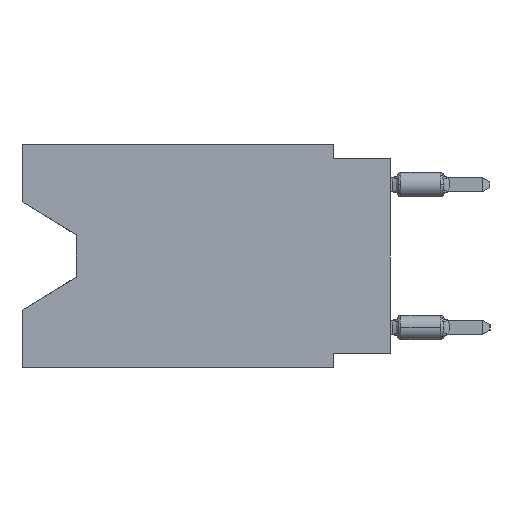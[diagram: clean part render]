
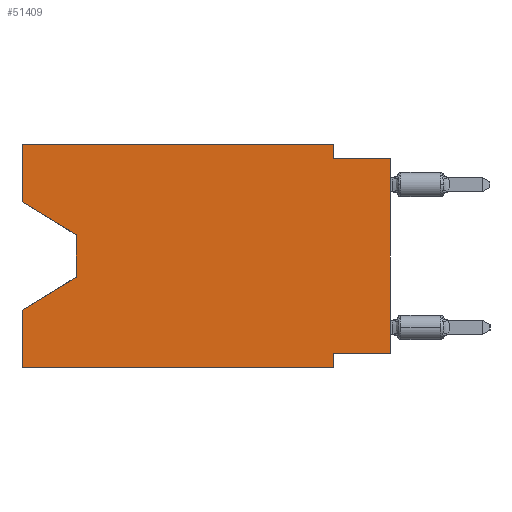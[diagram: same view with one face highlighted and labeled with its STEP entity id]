
A CAD part, left-side view. The second image highlights one B-rep face of the part: STEP entity #51409.
In plain terms, the highlighted planar face has unit normal (-1, 0, 0).
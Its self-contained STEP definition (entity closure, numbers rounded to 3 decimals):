
#362 = CARTESIAN_POINT ( 'NONE',  ( 0., 2.54, 0. ) ) ;
#564 = CARTESIAN_POINT ( 'NONE',  ( 0., 13.97, -5.893 ) ) ;
#1791 = DIRECTION ( 'NONE',  ( 0., -0.855, -0.519 ) ) ;
#2002 = EDGE_CURVE ( 'NONE', #8974, #5539, #24161, .T. ) ;
#2379 = EDGE_CURVE ( 'NONE', #8974, #27087, #26984, .T. ) ;
#2453 = VERTEX_POINT ( 'NONE', #19814 ) ;
#2467 = CARTESIAN_POINT ( 'NONE',  ( 0., 13.97, -4.013 ) ) ;
#2763 = DIRECTION ( 'NONE',  ( 0., 0., -1. ) ) ;
#2784 = ORIENTED_EDGE ( 'NONE', *, *, #38154, .F. ) ;
#3502 = ORIENTED_EDGE ( 'NONE', *, *, #9536, .F. ) ;
#4378 = CARTESIAN_POINT ( 'NONE',  ( 0., 2.54, -0.635 ) ) ;
#5166 = EDGE_CURVE ( 'NONE', #48027, #5539, #48782, .T. ) ;
#5539 = VERTEX_POINT ( 'NONE', #5601 ) ;
#5601 = CARTESIAN_POINT ( 'NONE',  ( 0., 16.383, -7.36 ) ) ;
#5624 = EDGE_LOOP ( 'NONE', ( #32298, #48143, #23040, #52216, #23704, #2784, #46701, #49892, #18983, #21154, #3502, #42232 ) ) ;
#6196 = VECTOR ( 'NONE', #33832, 1000. ) ;
#6949 = PLANE ( 'NONE',  #12384 ) ;
#7338 = VERTEX_POINT ( 'NONE', #50632 ) ;
#8920 = VECTOR ( 'NONE', #41881, 1000. ) ;
#8974 = VERTEX_POINT ( 'NONE', #37613 ) ;
#9085 = LINE ( 'NONE', #53320, #50934 ) ;
#9536 = EDGE_CURVE ( 'NONE', #7338, #35904, #38105, .T. ) ;
#11016 = DIRECTION ( 'NONE',  ( 0., 0., 1. ) ) ;
#12230 = CARTESIAN_POINT ( 'NONE',  ( 0., 13.97, -4.013 ) ) ;
#12384 = AXIS2_PLACEMENT_3D ( 'NONE', #55772, #50924, #42078 ) ;
#12525 = DIRECTION ( 'NONE',  ( 0., -1., 0. ) ) ;
#12752 = VECTOR ( 'NONE', #2763, 1000. ) ;
#13289 = CARTESIAN_POINT ( 'NONE',  ( 0., 16.383, -2.546 ) ) ;
#13306 = VERTEX_POINT ( 'NONE', #49402 ) ;
#14457 = CARTESIAN_POINT ( 'NONE',  ( 0., 16.383, 0. ) ) ;
#16087 = FACE_OUTER_BOUND ( 'NONE', #5624, .T. ) ;
#16602 = EDGE_CURVE ( 'NONE', #13306, #50716, #53113, .T. ) ;
#18411 = CARTESIAN_POINT ( 'NONE',  ( 0., 16.383, -9.906 ) ) ;
#18584 = VECTOR ( 'NONE', #12525, 1000. ) ;
#18983 = ORIENTED_EDGE ( 'NONE', *, *, #25957, .F. ) ;
#19137 = EDGE_CURVE ( 'NONE', #20633, #7338, #9085, .T. ) ;
#19209 = LINE ( 'NONE', #23770, #49213 ) ;
#19814 = CARTESIAN_POINT ( 'NONE',  ( 0., 0., -0.635 ) ) ;
#19903 = CARTESIAN_POINT ( 'NONE',  ( 0., 2.54, -9.906 ) ) ;
#20181 = EDGE_CURVE ( 'NONE', #13306, #2453, #43917, .T. ) ;
#20633 = VERTEX_POINT ( 'NONE', #13289 ) ;
#21119 = LINE ( 'NONE', #51641, #18584 ) ;
#21154 = ORIENTED_EDGE ( 'NONE', *, *, #41124, .F. ) ;
#21424 = CARTESIAN_POINT ( 'NONE',  ( 0., 2.54, -9.271 ) ) ;
#23040 = ORIENTED_EDGE ( 'NONE', *, *, #5166, .T. ) ;
#23704 = ORIENTED_EDGE ( 'NONE', *, *, #2379, .T. ) ;
#23770 = CARTESIAN_POINT ( 'NONE',  ( 0., 16.383, -2.546 ) ) ;
#24161 = LINE ( 'NONE', #14457, #25848 ) ;
#24461 = CARTESIAN_POINT ( 'NONE',  ( 0., 2.54, 0. ) ) ;
#25848 = VECTOR ( 'NONE', #11016, 1000. ) ;
#25957 = EDGE_CURVE ( 'NONE', #28882, #2453, #21119, .T. ) ;
#26522 = CARTESIAN_POINT ( 'NONE',  ( 0., 0., 0. ) ) ;
#26984 = LINE ( 'NONE', #18411, #54101 ) ;
#27087 = VERTEX_POINT ( 'NONE', #27353 ) ;
#27353 = CARTESIAN_POINT ( 'NONE',  ( 0., 2.54, -9.906 ) ) ;
#28882 = VERTEX_POINT ( 'NONE', #4378 ) ;
#30249 = LINE ( 'NONE', #12230, #34576 ) ;
#30517 = DIRECTION ( 'NONE',  ( 0., 0., -1. ) ) ;
#31356 = DIRECTION ( 'NONE',  ( 0., 0., 1. ) ) ;
#32213 = VERTEX_POINT ( 'NONE', #2467 ) ;
#32298 = ORIENTED_EDGE ( 'NONE', *, *, #54165, .T. ) ;
#33371 = VECTOR ( 'NONE', #35670, 1000. ) ;
#33832 = DIRECTION ( 'NONE',  ( 0., -1., 0. ) ) ;
#34576 = VECTOR ( 'NONE', #30517, 1000. ) ;
#35670 = DIRECTION ( 'NONE',  ( 0., 0.855, -0.519 ) ) ;
#35904 = VERTEX_POINT ( 'NONE', #362 ) ;
#36824 = CARTESIAN_POINT ( 'NONE',  ( 0., 0., -9.271 ) ) ;
#37613 = CARTESIAN_POINT ( 'NONE',  ( 0., 16.383, -9.906 ) ) ;
#37931 = EDGE_CURVE ( 'NONE', #32213, #48027, #30249, .T. ) ;
#38105 = LINE ( 'NONE', #55519, #6196 ) ;
#38154 = EDGE_CURVE ( 'NONE', #50716, #27087, #45303, .T. ) ;
#38707 = LINE ( 'NONE', #24461, #12752 ) ;
#39623 = DIRECTION ( 'NONE',  ( 0., 0., 1. ) ) ;
#41124 = EDGE_CURVE ( 'NONE', #35904, #28882, #38707, .T. ) ;
#41881 = DIRECTION ( 'NONE',  ( 0., 0., -1. ) ) ;
#42078 = DIRECTION ( 'NONE',  ( 0., 0., -1. ) ) ;
#42232 = ORIENTED_EDGE ( 'NONE', *, *, #19137, .F. ) ;
#43917 = LINE ( 'NONE', #26522, #53785 ) ;
#44373 = DIRECTION ( 'NONE',  ( 0., -1., 0. ) ) ;
#44499 = CARTESIAN_POINT ( 'NONE',  ( 0., 13.97, -5.893 ) ) ;
#45303 = LINE ( 'NONE', #19903, #8920 ) ;
#46701 = ORIENTED_EDGE ( 'NONE', *, *, #16602, .F. ) ;
#48027 = VERTEX_POINT ( 'NONE', #564 ) ;
#48143 = ORIENTED_EDGE ( 'NONE', *, *, #37931, .T. ) ;
#48782 = LINE ( 'NONE', #44499, #33371 ) ;
#49114 = DIRECTION ( 'NONE',  ( 0., 1., 0. ) ) ;
#49213 = VECTOR ( 'NONE', #1791, 1000. ) ;
#49402 = CARTESIAN_POINT ( 'NONE',  ( 0., 0., -9.271 ) ) ;
#49892 = ORIENTED_EDGE ( 'NONE', *, *, #20181, .T. ) ;
#50632 = CARTESIAN_POINT ( 'NONE',  ( 0., 16.383, 0. ) ) ;
#50716 = VERTEX_POINT ( 'NONE', #21424 ) ;
#50924 = DIRECTION ( 'NONE',  ( 1., 0., 0. ) ) ;
#50934 = VECTOR ( 'NONE', #39623, 1000. ) ;
#51409 = ADVANCED_FACE ( 'NONE', ( #16087 ), #6949, .F. ) ;
#51641 = CARTESIAN_POINT ( 'NONE',  ( 0., 0., -0.635 ) ) ;
#52216 = ORIENTED_EDGE ( 'NONE', *, *, #2002, .F. ) ;
#53113 = LINE ( 'NONE', #36824, #54516 ) ;
#53320 = CARTESIAN_POINT ( 'NONE',  ( 0., 16.383, 0. ) ) ;
#53785 = VECTOR ( 'NONE', #31356, 1000. ) ;
#54101 = VECTOR ( 'NONE', #44373, 1000. ) ;
#54165 = EDGE_CURVE ( 'NONE', #20633, #32213, #19209, .T. ) ;
#54516 = VECTOR ( 'NONE', #49114, 1000. ) ;
#55519 = CARTESIAN_POINT ( 'NONE',  ( 0., 16.383, 0. ) ) ;
#55772 = CARTESIAN_POINT ( 'NONE',  ( 0., 16.383, 0. ) ) ;
